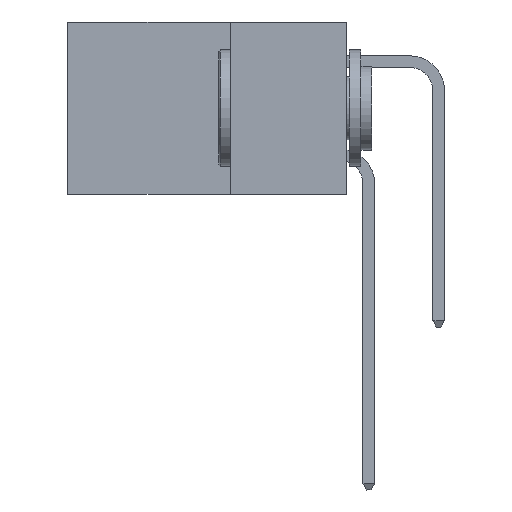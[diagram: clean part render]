
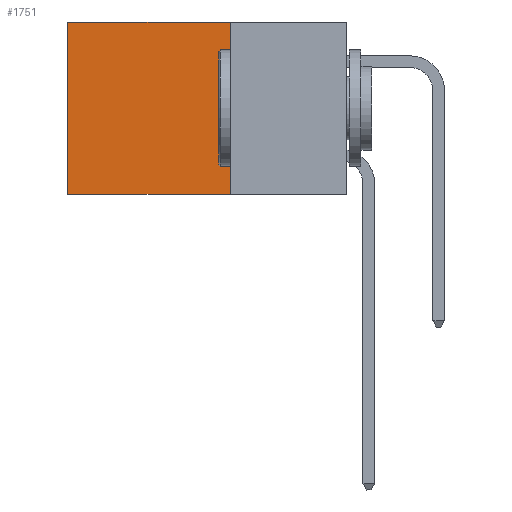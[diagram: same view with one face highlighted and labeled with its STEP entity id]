
A CAD part, left-side view. The second image highlights one B-rep face of the part: STEP entity #1751.
In plain terms, the highlighted planar face has unit normal (-1, 0, 0).
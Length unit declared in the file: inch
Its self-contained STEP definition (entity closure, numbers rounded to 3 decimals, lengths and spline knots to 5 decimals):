
#29 = CARTESIAN_POINT ( 'NONE',  ( 0.2875, 0.25, 0. ) ) ;
#60 = CARTESIAN_POINT ( 'NONE',  ( 0.2875, 0.25, -0.37 ) ) ;
#1133 = EDGE_LOOP ( 'NONE', ( #9841, #9949, #10018, #10161 ) ) ;
#1386 = DIRECTION ( 'NONE',  ( 0., 0., -1. ) ) ;
#1751 = ADVANCED_FACE ( 'NONE', ( #9470 ), #10423, .F. ) ;
#1883 = VECTOR ( 'NONE', #13107, 39.37008 ) ;
#2471 = EDGE_CURVE ( 'NONE', #6043, #11134, #2596, .T. ) ;
#2596 = LINE ( 'NONE', #29, #5317 ) ;
#2790 = EDGE_CURVE ( 'NONE', #6043, #7058, #11615, .T. ) ;
#2861 = DIRECTION ( 'NONE',  ( 0., 0., -1. ) ) ;
#2943 = CARTESIAN_POINT ( 'NONE',  ( 0.2875, 0.6, -0.37 ) ) ;
#3584 = VECTOR ( 'NONE', #10778, 39.37008 ) ;
#3877 = EDGE_CURVE ( 'NONE', #11134, #5232, #4320, .T. ) ;
#4320 = LINE ( 'NONE', #12946, #1883 ) ;
#4566 = VECTOR ( 'NONE', #2861, 39.37008 ) ;
#4609 = AXIS2_PLACEMENT_3D ( 'NONE', #10096, #9894, #9834 ) ;
#5200 = LINE ( 'NONE', #8955, #4566 ) ;
#5232 = VERTEX_POINT ( 'NONE', #2943 ) ;
#5317 = VECTOR ( 'NONE', #1386, 39.37008 ) ;
#5781 = CARTESIAN_POINT ( 'NONE',  ( 0.2875, 0.25, 0. ) ) ;
#6043 = VERTEX_POINT ( 'NONE', #5781 ) ;
#7058 = VERTEX_POINT ( 'NONE', #9439 ) ;
#8955 = CARTESIAN_POINT ( 'NONE',  ( 0.2875, 0.6, 0. ) ) ;
#8970 = EDGE_CURVE ( 'NONE', #7058, #5232, #5200, .T. ) ;
#9439 = CARTESIAN_POINT ( 'NONE',  ( 0.2875, 0.6, 0. ) ) ;
#9470 = FACE_OUTER_BOUND ( 'NONE', #1133, .T. ) ;
#9834 = DIRECTION ( 'NONE',  ( 0., 0., -1. ) ) ;
#9841 = ORIENTED_EDGE ( 'NONE', *, *, #8970, .T. ) ;
#9894 = DIRECTION ( 'NONE',  ( 1., 0., 0. ) ) ;
#9949 = ORIENTED_EDGE ( 'NONE', *, *, #3877, .F. ) ;
#10018 = ORIENTED_EDGE ( 'NONE', *, *, #2471, .F. ) ;
#10096 = CARTESIAN_POINT ( 'NONE',  ( 0.2875, 0.25, 0. ) ) ;
#10161 = ORIENTED_EDGE ( 'NONE', *, *, #2790, .T. ) ;
#10423 = PLANE ( 'NONE',  #4609 ) ;
#10456 = CARTESIAN_POINT ( 'NONE',  ( 0.2875, 0.25, 0. ) ) ;
#10778 = DIRECTION ( 'NONE',  ( 0., 1., 0. ) ) ;
#11134 = VERTEX_POINT ( 'NONE', #60 ) ;
#11615 = LINE ( 'NONE', #10456, #3584 ) ;
#12946 = CARTESIAN_POINT ( 'NONE',  ( 0.2875, 0.25, -0.37 ) ) ;
#13107 = DIRECTION ( 'NONE',  ( 0., 1., 0. ) ) ;
